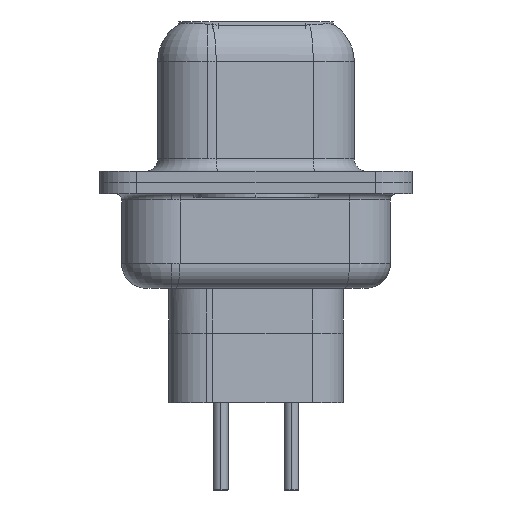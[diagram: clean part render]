
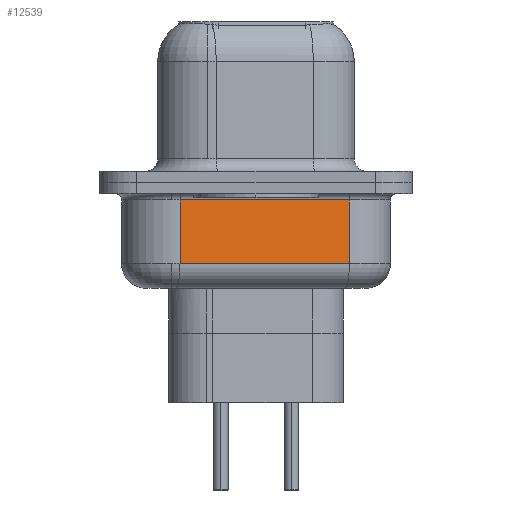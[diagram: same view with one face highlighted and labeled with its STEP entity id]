
A CAD part, left-side view. The second image highlights one B-rep face of the part: STEP entity #12539.
In plain terms, the highlighted planar face has unit normal (-0.985, -0.174, 0).
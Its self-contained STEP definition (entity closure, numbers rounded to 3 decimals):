
#1262 = CARTESIAN_POINT ( 'NONE',  ( 4.049, -3.747, -0.7 ) ) ;
#1847 = CARTESIAN_POINT ( 'NONE',  ( 2.85, 3.053, -4.25 ) ) ;
#1917 = DIRECTION ( 'NONE',  ( 0.985, 0.174, 0. ) ) ;
#3549 = CARTESIAN_POINT ( 'NONE',  ( 2.85, 3.053, -0.7 ) ) ;
#3821 = LINE ( 'NONE', #3549, #9783 ) ;
#5787 = LINE ( 'NONE', #1847, #21773 ) ;
#6325 = DIRECTION ( 'NONE',  ( 0., 0., 1. ) ) ;
#6388 = PLANE ( 'NONE',  #12124 ) ;
#6649 = EDGE_CURVE ( 'NONE', #26257, #14719, #3821, .T. ) ;
#7781 = CARTESIAN_POINT ( 'NONE',  ( 2.85, 3.053, -3.25 ) ) ;
#8673 = CARTESIAN_POINT ( 'NONE',  ( 2.85, 3.053, -4.25 ) ) ;
#9783 = VECTOR ( 'NONE', #21092, 1000. ) ;
#10237 = EDGE_LOOP ( 'NONE', ( #14562, #16956, #11968, #27598 ) ) ;
#10261 = FACE_OUTER_BOUND ( 'NONE', #10237, .T. ) ;
#10453 = VERTEX_POINT ( 'NONE', #7781 ) ;
#11836 = VECTOR ( 'NONE', #12960, 1000. ) ;
#11968 = ORIENTED_EDGE ( 'NONE', *, *, #18268, .T. ) ;
#12124 = AXIS2_PLACEMENT_3D ( 'NONE', #8673, #1917, #19335 ) ;
#12539 = ADVANCED_FACE ( 'NONE', ( #10261 ), #6388, .F. ) ;
#12870 = DIRECTION ( 'NONE',  ( 0., 0., 1. ) ) ;
#12960 = DIRECTION ( 'NONE',  ( 0.174, -0.985, 0. ) ) ;
#13074 = EDGE_CURVE ( 'NONE', #10453, #14719, #5787, .T. ) ;
#14562 = ORIENTED_EDGE ( 'NONE', *, *, #13074, .F. ) ;
#14719 = VERTEX_POINT ( 'NONE', #16764 ) ;
#14960 = CARTESIAN_POINT ( 'NONE',  ( 2.85, 3.053, -3.25 ) ) ;
#16764 = CARTESIAN_POINT ( 'NONE',  ( 2.85, 3.053, -0.7 ) ) ;
#16956 = ORIENTED_EDGE ( 'NONE', *, *, #21342, .T. ) ;
#18268 = EDGE_CURVE ( 'NONE', #21643, #26257, #22060, .T. ) ;
#19335 = DIRECTION ( 'NONE',  ( -0.174, 0.985, 0. ) ) ;
#19712 = LINE ( 'NONE', #14960, #11836 ) ;
#21092 = DIRECTION ( 'NONE',  ( -0.174, 0.985, 0. ) ) ;
#21263 = CARTESIAN_POINT ( 'NONE',  ( 4.049, -3.747, -3.25 ) ) ;
#21342 = EDGE_CURVE ( 'NONE', #10453, #21643, #19712, .T. ) ;
#21643 = VERTEX_POINT ( 'NONE', #21263 ) ;
#21773 = VECTOR ( 'NONE', #6325, 1000. ) ;
#22060 = LINE ( 'NONE', #28230, #23678 ) ;
#23678 = VECTOR ( 'NONE', #12870, 1000. ) ;
#26257 = VERTEX_POINT ( 'NONE', #1262 ) ;
#27598 = ORIENTED_EDGE ( 'NONE', *, *, #6649, .T. ) ;
#28230 = CARTESIAN_POINT ( 'NONE',  ( 4.049, -3.747, -4.25 ) ) ;
